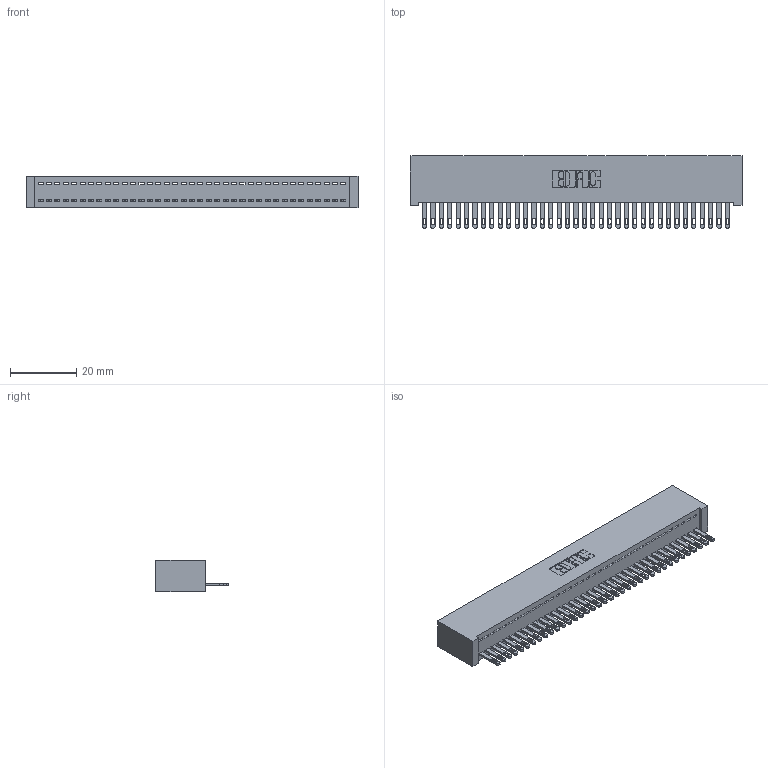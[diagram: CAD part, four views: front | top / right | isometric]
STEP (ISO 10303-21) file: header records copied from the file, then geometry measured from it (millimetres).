
FILE_DESCRIPTION (( 'STEP AP203' ), '1' );
FILE_NAME ('892-037-500-101.STEP', '2020-09-21T15:59:58', ( '' ), ( '' ), 'SwSTEP 2.0', 'SolidWorks 2020', '' );
FILE_SCHEMA (( 'CONFIG_CONTROL_DESIGN' ));
Length unit declared in the file: inch
Products named in the file (3): 892-037-500-101; 842 Part_Lugless; 345-292-001_345-293-100
Assembly tree (38 placements, depth 2):
  892-037-500-101
    842 Part_Lugless
    345-292-001_345-293-100  x37
Bounding box: 100.23 x 21.85 x 9.4 mm (x, y, z)
Volume: 9201.5 mm3; surface area: 13814.7 mm2
Topology: 38 solids, 38 shells, 2100 faces, 6491 edges, 4326 vertices
Faces by surface type: plane 1394, cylinder 706
Entity records: 22787 total; most frequent: CARTESIAN_POINT 3937, ORIENTED_EDGE 3910, DIRECTION 3325, EDGE_CURVE 1955, VECTOR 1831, LINE 1831, VERTEX_POINT 1302, AXIS2_PLACEMENT_3D 747
